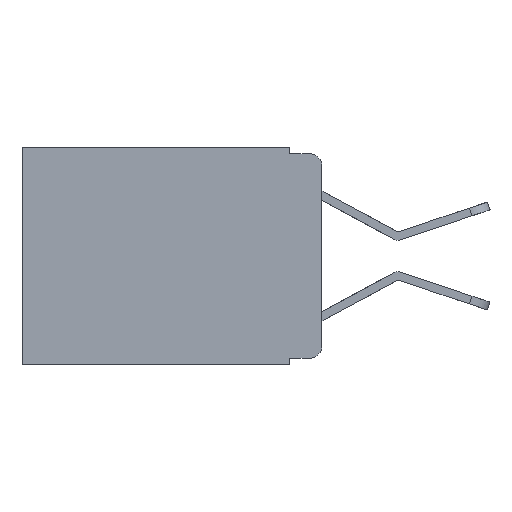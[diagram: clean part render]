
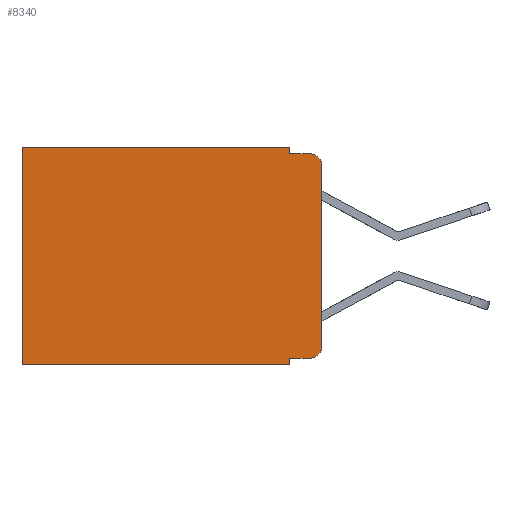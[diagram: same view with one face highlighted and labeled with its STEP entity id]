
A CAD part, left-side view. The second image highlights one B-rep face of the part: STEP entity #8340.
In plain terms, the highlighted planar face has unit normal (-1, 0, 0).
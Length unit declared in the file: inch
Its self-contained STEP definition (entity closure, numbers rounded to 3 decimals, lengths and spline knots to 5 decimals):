
#134 = VECTOR ( 'NONE', #3006, 39.37008 ) ;
#352 = CARTESIAN_POINT ( 'NONE',  ( 0.298, 0.051, 0. ) ) ;
#509 = CARTESIAN_POINT ( 'NONE',  ( 0.298, 0.051, 0. ) ) ;
#533 = DIRECTION ( 'NONE',  ( 0., 0., -1. ) ) ;
#771 = CARTESIAN_POINT ( 'NONE',  ( 0.298, 0., -0.313 ) ) ;
#1145 = CARTESIAN_POINT ( 'NONE',  ( 0.298, 0.051, -0.343 ) ) ;
#1289 = LINE ( 'NONE', #11230, #12547 ) ;
#1339 = CARTESIAN_POINT ( 'NONE',  ( 0.298, 0., 0. ) ) ;
#1364 = DIRECTION ( 'NONE',  ( 0., 1., 0. ) ) ;
#1483 = ORIENTED_EDGE ( 'NONE', *, *, #4362, .F. ) ;
#1666 = CARTESIAN_POINT ( 'NONE',  ( 0.298, 0., -0.343 ) ) ;
#1944 = EDGE_CURVE ( 'NONE', #11237, #3857, #6856, .T. ) ;
#2023 = EDGE_LOOP ( 'NONE', ( #9687, #4486, #9351, #3285, #2615, #8095, #13303, #1483, #12678, #6674 ) ) ;
#2210 = VECTOR ( 'NONE', #5598, 39.37008 ) ;
#2257 = LINE ( 'NONE', #6577, #13289 ) ;
#2553 = LINE ( 'NONE', #13215, #2210 ) ;
#2596 = EDGE_CURVE ( 'NONE', #11237, #8074, #2257, .T. ) ;
#2615 = ORIENTED_EDGE ( 'NONE', *, *, #1944, .T. ) ;
#2764 = CARTESIAN_POINT ( 'NONE',  ( 0.298, 0.02, -0.333 ) ) ;
#2927 = EDGE_CURVE ( 'NONE', #12630, #10619, #14049, .T. ) ;
#3006 = DIRECTION ( 'NONE',  ( 0., 0., -1. ) ) ;
#3065 = VECTOR ( 'NONE', #5915, 39.37008 ) ;
#3078 = VECTOR ( 'NONE', #3132, 39.37008 ) ;
#3115 = VERTEX_POINT ( 'NONE', #10740 ) ;
#3132 = DIRECTION ( 'NONE',  ( 0., -1., 0. ) ) ;
#3257 = CIRCLE ( 'NONE', #8703, 0.02 ) ;
#3285 = ORIENTED_EDGE ( 'NONE', *, *, #2596, .F. ) ;
#3306 = EDGE_CURVE ( 'NONE', #5160, #5005, #3257, .T. ) ;
#3310 = CARTESIAN_POINT ( 'NONE',  ( 0.298, 0.473, 0. ) ) ;
#3419 = LINE ( 'NONE', #5123, #3078 ) ;
#3662 = EDGE_CURVE ( 'NONE', #3115, #12630, #3419, .T. ) ;
#3857 = VERTEX_POINT ( 'NONE', #3310 ) ;
#3987 = VECTOR ( 'NONE', #1364, 39.37008 ) ;
#4251 = AXIS2_PLACEMENT_3D ( 'NONE', #11372, #11370, #11343 ) ;
#4362 = EDGE_CURVE ( 'NONE', #3115, #8084, #6265, .T. ) ;
#4486 = ORIENTED_EDGE ( 'NONE', *, *, #3306, .T. ) ;
#5005 = VERTEX_POINT ( 'NONE', #10712 ) ;
#5095 = EDGE_CURVE ( 'NONE', #3857, #7834, #6107, .T. ) ;
#5123 = CARTESIAN_POINT ( 'NONE',  ( 0.298, 0.051, -0.333 ) ) ;
#5142 = PLANE ( 'NONE',  #10467 ) ;
#5160 = VERTEX_POINT ( 'NONE', #7148 ) ;
#5598 = DIRECTION ( 'NONE',  ( 0., -1., 0. ) ) ;
#5915 = DIRECTION ( 'NONE',  ( 0., 0., -1. ) ) ;
#5995 = DIRECTION ( 'NONE',  ( 0., 0., -1. ) ) ;
#6032 = DIRECTION ( 'NONE',  ( -1., 0., 0. ) ) ;
#6044 = CARTESIAN_POINT ( 'NONE',  ( 0.298, 0.02, -0.03 ) ) ;
#6073 = EDGE_CURVE ( 'NONE', #8084, #7834, #7849, .T. ) ;
#6107 = LINE ( 'NONE', #8038, #134 ) ;
#6125 = DIRECTION ( 'NONE',  ( 0., 0., -1. ) ) ;
#6192 = EDGE_CURVE ( 'NONE', #8074, #5005, #2553, .T. ) ;
#6265 = LINE ( 'NONE', #509, #3065 ) ;
#6577 = CARTESIAN_POINT ( 'NONE',  ( 0.298, 0.051, 0. ) ) ;
#6674 = ORIENTED_EDGE ( 'NONE', *, *, #2927, .T. ) ;
#6856 = LINE ( 'NONE', #1339, #3987 ) ;
#7148 = CARTESIAN_POINT ( 'NONE',  ( 0.298, 0., -0.03 ) ) ;
#7357 = DIRECTION ( 'NONE',  ( 1., 0., 0. ) ) ;
#7834 = VERTEX_POINT ( 'NONE', #8430 ) ;
#7849 = LINE ( 'NONE', #1666, #13082 ) ;
#8038 = CARTESIAN_POINT ( 'NONE',  ( 0.298, 0.473, 0. ) ) ;
#8074 = VERTEX_POINT ( 'NONE', #11107 ) ;
#8084 = VERTEX_POINT ( 'NONE', #1145 ) ;
#8095 = ORIENTED_EDGE ( 'NONE', *, *, #5095, .T. ) ;
#8105 = DIRECTION ( 'NONE',  ( 0., 1., 0. ) ) ;
#8340 = ADVANCED_FACE ( 'NONE', ( #9264 ), #5142, .F. ) ;
#8430 = CARTESIAN_POINT ( 'NONE',  ( 0.298, 0.473, -0.343 ) ) ;
#8703 = AXIS2_PLACEMENT_3D ( 'NONE', #6044, #6032, #5995 ) ;
#9264 = FACE_OUTER_BOUND ( 'NONE', #2023, .T. ) ;
#9351 = ORIENTED_EDGE ( 'NONE', *, *, #6192, .F. ) ;
#9687 = ORIENTED_EDGE ( 'NONE', *, *, #13808, .F. ) ;
#10467 = AXIS2_PLACEMENT_3D ( 'NONE', #12641, #7357, #533 ) ;
#10619 = VERTEX_POINT ( 'NONE', #771 ) ;
#10712 = CARTESIAN_POINT ( 'NONE',  ( 0.298, 0.02, -0.01 ) ) ;
#10740 = CARTESIAN_POINT ( 'NONE',  ( 0.298, 0.051, -0.333 ) ) ;
#11107 = CARTESIAN_POINT ( 'NONE',  ( 0.298, 0.051, -0.01 ) ) ;
#11230 = CARTESIAN_POINT ( 'NONE',  ( 0.298, 0., 0. ) ) ;
#11237 = VERTEX_POINT ( 'NONE', #352 ) ;
#11343 = DIRECTION ( 'NONE',  ( 0., 0., -1. ) ) ;
#11370 = DIRECTION ( 'NONE',  ( -1., 0., 0. ) ) ;
#11372 = CARTESIAN_POINT ( 'NONE',  ( 0.298, 0.02, -0.313 ) ) ;
#12271 = DIRECTION ( 'NONE',  ( 0., 0., -1. ) ) ;
#12547 = VECTOR ( 'NONE', #12271, 39.37008 ) ;
#12630 = VERTEX_POINT ( 'NONE', #2764 ) ;
#12641 = CARTESIAN_POINT ( 'NONE',  ( 0.298, 0., 0. ) ) ;
#12678 = ORIENTED_EDGE ( 'NONE', *, *, #3662, .T. ) ;
#13082 = VECTOR ( 'NONE', #8105, 39.37008 ) ;
#13215 = CARTESIAN_POINT ( 'NONE',  ( 0.298, 0.051, -0.01 ) ) ;
#13289 = VECTOR ( 'NONE', #6125, 39.37008 ) ;
#13303 = ORIENTED_EDGE ( 'NONE', *, *, #6073, .F. ) ;
#13808 = EDGE_CURVE ( 'NONE', #5160, #10619, #1289, .T. ) ;
#14049 = CIRCLE ( 'NONE', #4251, 0.02 ) ;
